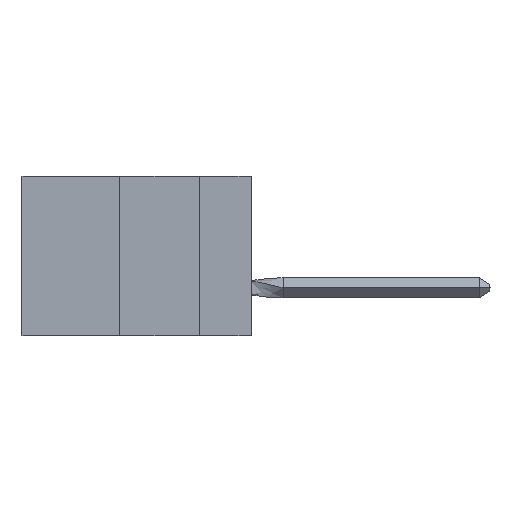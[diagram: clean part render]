
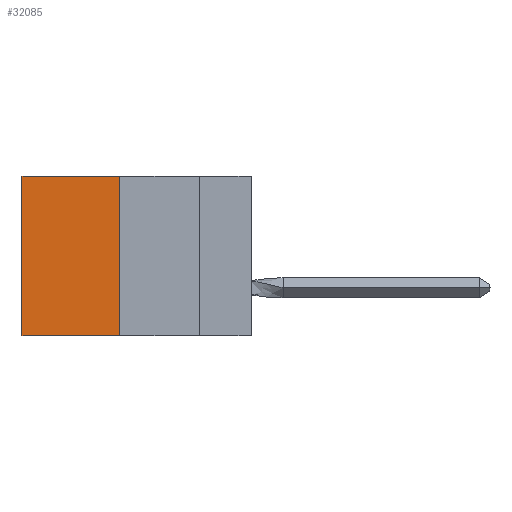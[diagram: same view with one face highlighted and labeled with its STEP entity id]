
A CAD part, left-side view. The second image highlights one B-rep face of the part: STEP entity #32085.
In plain terms, the highlighted planar face has unit normal (-1, 0, 0).
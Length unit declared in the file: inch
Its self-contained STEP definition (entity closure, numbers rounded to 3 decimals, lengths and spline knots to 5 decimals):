
#1214 = PLANE ( 'NONE',  #18144 ) ;
#1416 = VERTEX_POINT ( 'NONE', #33496 ) ;
#1558 = CARTESIAN_POINT ( 'NONE',  ( 0.305, 0.72, -0.5 ) ) ;
#1947 = DIRECTION ( 'NONE',  ( 0., 0., -1. ) ) ;
#2264 = EDGE_LOOP ( 'NONE', ( #35738, #10263, #17306, #28562 ) ) ;
#5877 = CARTESIAN_POINT ( 'NONE',  ( 0.305, 0.413, 0. ) ) ;
#6612 = EDGE_CURVE ( 'NONE', #8051, #37387, #12966, .T. ) ;
#6883 = CARTESIAN_POINT ( 'NONE',  ( 0.305, 0.413, -0.5 ) ) ;
#6932 = CARTESIAN_POINT ( 'NONE',  ( 0.305, 0.413, -0.5 ) ) ;
#8051 = VERTEX_POINT ( 'NONE', #5877 ) ;
#9963 = DIRECTION ( 'NONE',  ( 0., 0., -1. ) ) ;
#10263 = ORIENTED_EDGE ( 'NONE', *, *, #24397, .F. ) ;
#10810 = CARTESIAN_POINT ( 'NONE',  ( 0.305, 0.413, -0.5 ) ) ;
#11524 = LINE ( 'NONE', #6932, #31572 ) ;
#12521 = LINE ( 'NONE', #22387, #18461 ) ;
#12966 = LINE ( 'NONE', #30337, #19812 ) ;
#13313 = DIRECTION ( 'NONE',  ( 0., 1., 0. ) ) ;
#14937 = VERTEX_POINT ( 'NONE', #28638 ) ;
#17306 = ORIENTED_EDGE ( 'NONE', *, *, #6612, .F. ) ;
#18144 = AXIS2_PLACEMENT_3D ( 'NONE', #6883, #21685, #9963 ) ;
#18461 = VECTOR ( 'NONE', #13313, 39.37008 ) ;
#19812 = VECTOR ( 'NONE', #36236, 39.37008 ) ;
#21669 = LINE ( 'NONE', #1558, #23511 ) ;
#21685 = DIRECTION ( 'NONE',  ( 1., 0., 0. ) ) ;
#22387 = CARTESIAN_POINT ( 'NONE',  ( 0.305, 0.413, 0. ) ) ;
#23511 = VECTOR ( 'NONE', #1947, 39.37008 ) ;
#24397 = EDGE_CURVE ( 'NONE', #37387, #14937, #11524, .T. ) ;
#27364 = DIRECTION ( 'NONE',  ( 0., 1., 0. ) ) ;
#28148 = EDGE_CURVE ( 'NONE', #1416, #14937, #21669, .T. ) ;
#28562 = ORIENTED_EDGE ( 'NONE', *, *, #36097, .T. ) ;
#28638 = CARTESIAN_POINT ( 'NONE',  ( 0.305, 0.72, -0.5 ) ) ;
#30337 = CARTESIAN_POINT ( 'NONE',  ( 0.305, 0.413, -0.5 ) ) ;
#31572 = VECTOR ( 'NONE', #27364, 39.37008 ) ;
#32085 = ADVANCED_FACE ( 'NONE', ( #35638 ), #1214, .F. ) ;
#33496 = CARTESIAN_POINT ( 'NONE',  ( 0.305, 0.72, 0. ) ) ;
#35638 = FACE_OUTER_BOUND ( 'NONE', #2264, .T. ) ;
#35738 = ORIENTED_EDGE ( 'NONE', *, *, #28148, .T. ) ;
#36097 = EDGE_CURVE ( 'NONE', #8051, #1416, #12521, .T. ) ;
#36236 = DIRECTION ( 'NONE',  ( 0., 0., -1. ) ) ;
#37387 = VERTEX_POINT ( 'NONE', #10810 ) ;
